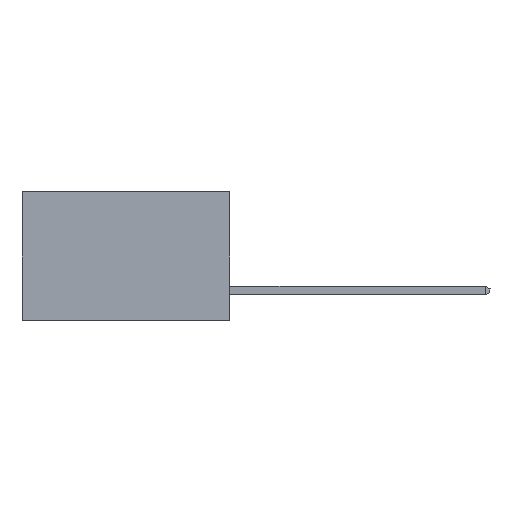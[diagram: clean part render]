
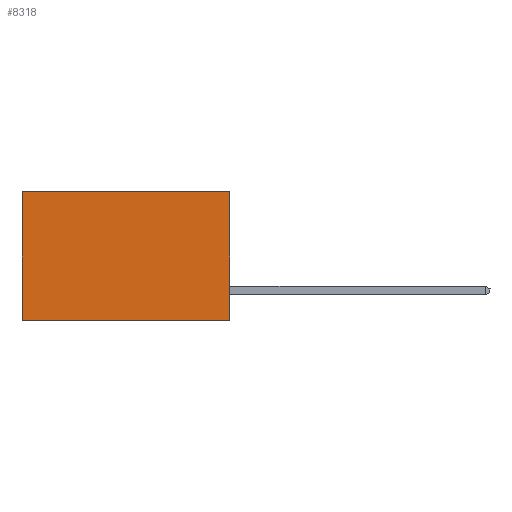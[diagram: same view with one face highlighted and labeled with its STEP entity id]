
A CAD part, left-side view. The second image highlights one B-rep face of the part: STEP entity #8318.
In plain terms, the highlighted planar face has unit normal (-1, 0, 0).
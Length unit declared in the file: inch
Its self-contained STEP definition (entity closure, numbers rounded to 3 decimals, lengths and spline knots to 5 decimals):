
#207 = CARTESIAN_POINT ( 'NONE',  ( 0.2615, 0.6, -0.37 ) ) ;
#307 = LINE ( 'NONE', #1603, #4512 ) ;
#986 = DIRECTION ( 'NONE',  ( 0., 0., -1. ) ) ;
#1386 = FACE_OUTER_BOUND ( 'NONE', #6603, .T. ) ;
#1401 = VERTEX_POINT ( 'NONE', #4660 ) ;
#1603 = CARTESIAN_POINT ( 'NONE',  ( 0.2615, 0., 0. ) ) ;
#1641 = DIRECTION ( 'NONE',  ( 0., 1., 0. ) ) ;
#1707 = ORIENTED_EDGE ( 'NONE', *, *, #6749, .T. ) ;
#2149 = EDGE_CURVE ( 'NONE', #5215, #1401, #307, .T. ) ;
#2309 = LINE ( 'NONE', #3164, #6150 ) ;
#2510 = ORIENTED_EDGE ( 'NONE', *, *, #2149, .T. ) ;
#2512 = VERTEX_POINT ( 'NONE', #207 ) ;
#2551 = VECTOR ( 'NONE', #986, 39.37008 ) ;
#2801 = DIRECTION ( 'NONE',  ( 1., 0., 0. ) ) ;
#3070 = DIRECTION ( 'NONE',  ( 0., 0., -1. ) ) ;
#3164 = CARTESIAN_POINT ( 'NONE',  ( 0.2615, 0.6, -0.37 ) ) ;
#3397 = CARTESIAN_POINT ( 'NONE',  ( 0.2615, 0., -0.37 ) ) ;
#3575 = AXIS2_PLACEMENT_3D ( 'NONE', #6905, #2801, #5542 ) ;
#3781 = LINE ( 'NONE', #5769, #2551 ) ;
#4370 = CARTESIAN_POINT ( 'NONE',  ( 0.2615, 0., 0. ) ) ;
#4512 = VECTOR ( 'NONE', #1641, 39.37008 ) ;
#4660 = CARTESIAN_POINT ( 'NONE',  ( 0.2615, 0.6, 0. ) ) ;
#5215 = VERTEX_POINT ( 'NONE', #4370 ) ;
#5440 = VERTEX_POINT ( 'NONE', #8538 ) ;
#5478 = DIRECTION ( 'NONE',  ( 0., 1., 0. ) ) ;
#5542 = DIRECTION ( 'NONE',  ( 0., 0., -1. ) ) ;
#5769 = CARTESIAN_POINT ( 'NONE',  ( 0.2615, 0., -0.37 ) ) ;
#5938 = EDGE_CURVE ( 'NONE', #5440, #2512, #7483, .T. ) ;
#6150 = VECTOR ( 'NONE', #3070, 39.37008 ) ;
#6571 = VECTOR ( 'NONE', #5478, 39.37008 ) ;
#6603 = EDGE_LOOP ( 'NONE', ( #1707, #7349, #6607, #2510 ) ) ;
#6607 = ORIENTED_EDGE ( 'NONE', *, *, #6802, .F. ) ;
#6749 = EDGE_CURVE ( 'NONE', #1401, #2512, #2309, .T. ) ;
#6802 = EDGE_CURVE ( 'NONE', #5215, #5440, #3781, .T. ) ;
#6905 = CARTESIAN_POINT ( 'NONE',  ( 0.2615, 0., -0.37 ) ) ;
#7349 = ORIENTED_EDGE ( 'NONE', *, *, #5938, .F. ) ;
#7483 = LINE ( 'NONE', #3397, #6571 ) ;
#7551 = PLANE ( 'NONE',  #3575 ) ;
#8318 = ADVANCED_FACE ( 'NONE', ( #1386 ), #7551, .F. ) ;
#8538 = CARTESIAN_POINT ( 'NONE',  ( 0.2615, 0., -0.37 ) ) ;
